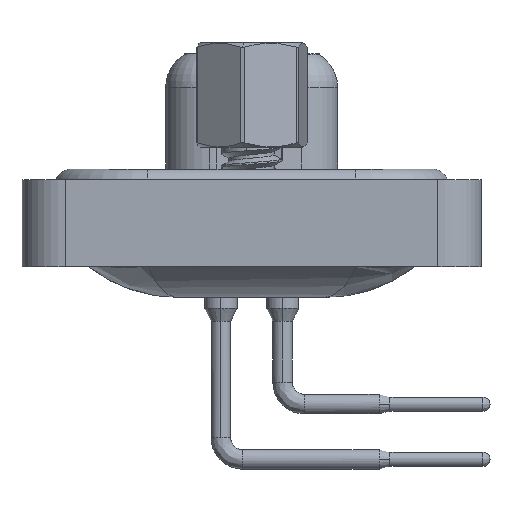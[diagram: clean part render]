
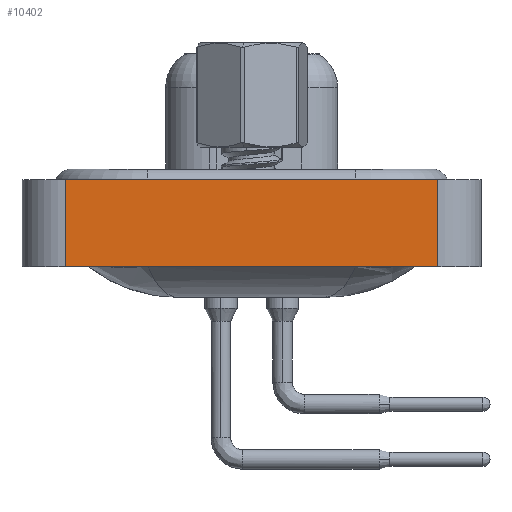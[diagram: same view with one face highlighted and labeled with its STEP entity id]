
A CAD part, left-side view. The second image highlights one B-rep face of the part: STEP entity #10402.
In plain terms, the highlighted planar face has unit normal (-1, 0, 0).
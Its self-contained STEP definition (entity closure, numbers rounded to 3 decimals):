
#108 = CARTESIAN_POINT ( 'NONE',  ( -7.285, -8.55, 0.4 ) ) ;
#166 = CARTESIAN_POINT ( 'NONE',  ( -7.285, 8.55, -3.6 ) ) ;
#962 = CARTESIAN_POINT ( 'NONE',  ( -7.285, -8.55, -3.6 ) ) ;
#1968 = CARTESIAN_POINT ( 'NONE',  ( -7.285, -8.55, -3.6 ) ) ;
#1994 = CARTESIAN_POINT ( 'NONE',  ( -7.285, 8.55, 0.4 ) ) ;
#2010 = ORIENTED_EDGE ( 'NONE', *, *, #18035, .F. ) ;
#2597 = VERTEX_POINT ( 'NONE', #1968 ) ;
#4756 = ORIENTED_EDGE ( 'NONE', *, *, #19933, .F. ) ;
#5157 = EDGE_LOOP ( 'NONE', ( #20629, #2010, #4756, #5686 ) ) ;
#5686 = ORIENTED_EDGE ( 'NONE', *, *, #12744, .T. ) ;
#5844 = DIRECTION ( 'NONE',  ( 0., -1., 0. ) ) ;
#6445 = VERTEX_POINT ( 'NONE', #1994 ) ;
#7035 = DIRECTION ( 'NONE',  ( 0., 0., 1. ) ) ;
#7076 = DIRECTION ( 'NONE',  ( 0., -1., 0. ) ) ;
#7756 = CARTESIAN_POINT ( 'NONE',  ( -7.285, 8.55, -3.6 ) ) ;
#7804 = LINE ( 'NONE', #11109, #9290 ) ;
#7994 = LINE ( 'NONE', #7756, #10249 ) ;
#9290 = VECTOR ( 'NONE', #5844, 1000. ) ;
#9814 = DIRECTION ( 'NONE',  ( 0., 0., 1. ) ) ;
#9860 = CARTESIAN_POINT ( 'NONE',  ( -7.285, -8.55, -3.6 ) ) ;
#10249 = VECTOR ( 'NONE', #9814, 1000. ) ;
#10402 = ADVANCED_FACE ( 'NONE', ( #17078 ), #20750, .T. ) ;
#10844 = VECTOR ( 'NONE', #7035, 1000. ) ;
#11109 = CARTESIAN_POINT ( 'NONE',  ( -7.285, -8.55, 0.4 ) ) ;
#12744 = EDGE_CURVE ( 'NONE', #17073, #2597, #23479, .T. ) ;
#13526 = DIRECTION ( 'NONE',  ( -1., 0., 0. ) ) ;
#14362 = VERTEX_POINT ( 'NONE', #108 ) ;
#14583 = VECTOR ( 'NONE', #7076, 1000. ) ;
#14856 = AXIS2_PLACEMENT_3D ( 'NONE', #9860, #13526, #15232 ) ;
#15232 = DIRECTION ( 'NONE',  ( 0., 0., 1. ) ) ;
#17073 = VERTEX_POINT ( 'NONE', #166 ) ;
#17078 = FACE_OUTER_BOUND ( 'NONE', #5157, .T. ) ;
#17823 = LINE ( 'NONE', #19657, #10844 ) ;
#18035 = EDGE_CURVE ( 'NONE', #6445, #14362, #7804, .T. ) ;
#18338 = EDGE_CURVE ( 'NONE', #2597, #14362, #17823, .T. ) ;
#19657 = CARTESIAN_POINT ( 'NONE',  ( -7.285, -8.55, -3.6 ) ) ;
#19933 = EDGE_CURVE ( 'NONE', #17073, #6445, #7994, .T. ) ;
#20629 = ORIENTED_EDGE ( 'NONE', *, *, #18338, .T. ) ;
#20750 = PLANE ( 'NONE',  #14856 ) ;
#23479 = LINE ( 'NONE', #962, #14583 ) ;
